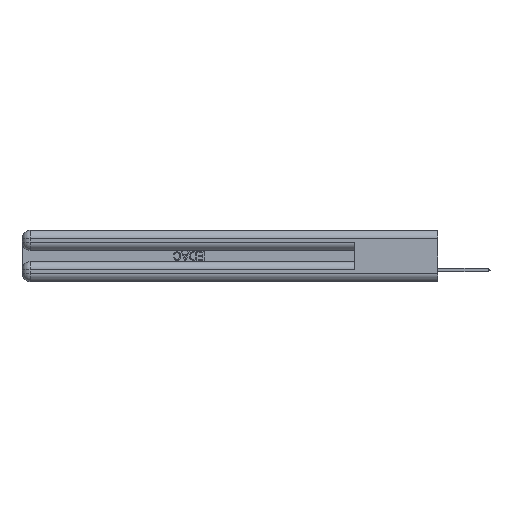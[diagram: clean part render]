
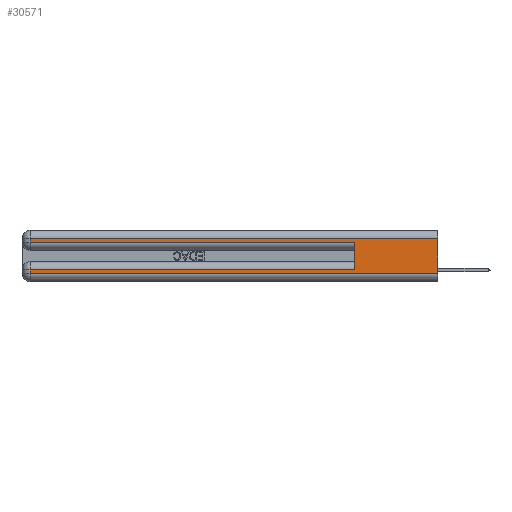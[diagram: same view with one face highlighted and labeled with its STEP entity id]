
A CAD part, left-side view. The second image highlights one B-rep face of the part: STEP entity #30571.
In plain terms, the highlighted planar face has unit normal (-1, 0, 0).
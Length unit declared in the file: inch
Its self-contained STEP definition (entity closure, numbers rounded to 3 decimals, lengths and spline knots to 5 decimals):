
#95 = VECTOR ( 'NONE', #26432, 39.37008 ) ;
#1609 = VERTEX_POINT ( 'NONE', #29147 ) ;
#1944 = DIRECTION ( 'NONE',  ( 0., 0., 1. ) ) ;
#2516 = LINE ( 'NONE', #33117, #41497 ) ;
#3719 = EDGE_CURVE ( 'NONE', #3980, #8936, #18678, .T. ) ;
#3980 = VERTEX_POINT ( 'NONE', #30022 ) ;
#4600 = DIRECTION ( 'NONE',  ( 0., 1., 0. ) ) ;
#4933 = CARTESIAN_POINT ( 'NONE',  ( 0., 0., 0.06 ) ) ;
#6316 = ORIENTED_EDGE ( 'NONE', *, *, #44853, .T. ) ;
#6762 = ORIENTED_EDGE ( 'NONE', *, *, #10322, .T. ) ;
#6865 = ORIENTED_EDGE ( 'NONE', *, *, #19535, .T. ) ;
#7500 = DIRECTION ( 'NONE',  ( 0., -1., 0. ) ) ;
#8032 = VERTEX_POINT ( 'NONE', #39500 ) ;
#8234 = DIRECTION ( 'NONE',  ( 0., 0., -1. ) ) ;
#8912 = ORIENTED_EDGE ( 'NONE', *, *, #9733, .T. ) ;
#8936 = VERTEX_POINT ( 'NONE', #36138 ) ;
#9104 = VECTOR ( 'NONE', #4600, 39.37008 ) ;
#9733 = EDGE_CURVE ( 'NONE', #8032, #42723, #23726, .T. ) ;
#10322 = EDGE_CURVE ( 'NONE', #42344, #1609, #27430, .T. ) ;
#11718 = CARTESIAN_POINT ( 'NONE',  ( 0., 0.6, 0.085 ) ) ;
#12474 = CARTESIAN_POINT ( 'NONE',  ( 0., 0., 0.37 ) ) ;
#14297 = LINE ( 'NONE', #22458, #20802 ) ;
#14935 = ORIENTED_EDGE ( 'NONE', *, *, #3719, .T. ) ;
#15551 = VECTOR ( 'NONE', #15946, 39.37008 ) ;
#15946 = DIRECTION ( 'NONE',  ( 0., 0., -1. ) ) ;
#16464 = CARTESIAN_POINT ( 'NONE',  ( 0., 0., 0.06 ) ) ;
#18678 = LINE ( 'NONE', #38413, #30072 ) ;
#19535 = EDGE_CURVE ( 'NONE', #1609, #21845, #23922, .T. ) ;
#19687 = CARTESIAN_POINT ( 'NONE',  ( 0., 2.94, 0.37 ) ) ;
#20802 = VECTOR ( 'NONE', #1944, 39.37008 ) ;
#21104 = AXIS2_PLACEMENT_3D ( 'NONE', #28635, #36262, #8234 ) ;
#21350 = VERTEX_POINT ( 'NONE', #11718 ) ;
#21673 = PLANE ( 'NONE',  #21104 ) ;
#21845 = VERTEX_POINT ( 'NONE', #4933 ) ;
#22373 = DIRECTION ( 'NONE',  ( 0., 1., 0. ) ) ;
#22458 = CARTESIAN_POINT ( 'NONE',  ( 0., 0.6, 0.145 ) ) ;
#23205 = ORIENTED_EDGE ( 'NONE', *, *, #40434, .F. ) ;
#23284 = EDGE_CURVE ( 'NONE', #21350, #42344, #2516, .T. ) ;
#23726 = LINE ( 'NONE', #25787, #9104 ) ;
#23922 = LINE ( 'NONE', #16464, #26622 ) ;
#24371 = LINE ( 'NONE', #33530, #95 ) ;
#25787 = CARTESIAN_POINT ( 'NONE',  ( 0., 0., 0.31 ) ) ;
#26352 = FACE_OUTER_BOUND ( 'NONE', #33024, .T. ) ;
#26432 = DIRECTION ( 'NONE',  ( 0., 0., -1. ) ) ;
#26622 = VECTOR ( 'NONE', #7500, 39.37008 ) ;
#26859 = CARTESIAN_POINT ( 'NONE',  ( 0., 2.94, 0.085 ) ) ;
#27430 = LINE ( 'NONE', #19687, #31220 ) ;
#28310 = CARTESIAN_POINT ( 'NONE',  ( 0., 2.94, 0.31 ) ) ;
#28635 = CARTESIAN_POINT ( 'NONE',  ( 0., 0., 0.37 ) ) ;
#29147 = CARTESIAN_POINT ( 'NONE',  ( 0., 2.94, 0.06 ) ) ;
#30022 = CARTESIAN_POINT ( 'NONE',  ( 0., 2.94, 0.285 ) ) ;
#30072 = VECTOR ( 'NONE', #34328, 39.37008 ) ;
#30571 = ADVANCED_FACE ( 'NONE', ( #26352 ), #21673, .F. ) ;
#31220 = VECTOR ( 'NONE', #36569, 39.37008 ) ;
#32533 = ORIENTED_EDGE ( 'NONE', *, *, #33287, .F. ) ;
#33024 = EDGE_LOOP ( 'NONE', ( #32533, #8912, #6316, #14935, #23205, #43644, #6762, #6865 ) ) ;
#33117 = CARTESIAN_POINT ( 'NONE',  ( 0., 0., 0.085 ) ) ;
#33287 = EDGE_CURVE ( 'NONE', #8032, #21845, #42630, .T. ) ;
#33530 = CARTESIAN_POINT ( 'NONE',  ( 0., 2.94, 0.37 ) ) ;
#34328 = DIRECTION ( 'NONE',  ( 0., -1., 0. ) ) ;
#36138 = CARTESIAN_POINT ( 'NONE',  ( 0., 0.6, 0.285 ) ) ;
#36262 = DIRECTION ( 'NONE',  ( 1., 0., 0. ) ) ;
#36569 = DIRECTION ( 'NONE',  ( 0., 0., -1. ) ) ;
#38413 = CARTESIAN_POINT ( 'NONE',  ( 0., 0., 0.285 ) ) ;
#39500 = CARTESIAN_POINT ( 'NONE',  ( 0., 0., 0.31 ) ) ;
#40434 = EDGE_CURVE ( 'NONE', #21350, #8936, #14297, .T. ) ;
#41497 = VECTOR ( 'NONE', #22373, 39.37008 ) ;
#42344 = VERTEX_POINT ( 'NONE', #26859 ) ;
#42630 = LINE ( 'NONE', #12474, #15551 ) ;
#42723 = VERTEX_POINT ( 'NONE', #28310 ) ;
#43644 = ORIENTED_EDGE ( 'NONE', *, *, #23284, .T. ) ;
#44853 = EDGE_CURVE ( 'NONE', #42723, #3980, #24371, .T. ) ;
